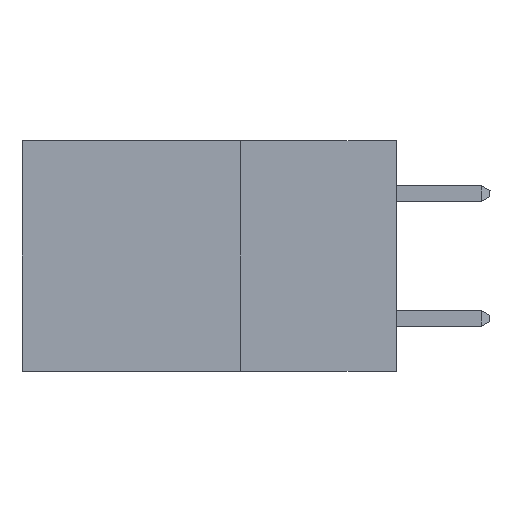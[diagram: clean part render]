
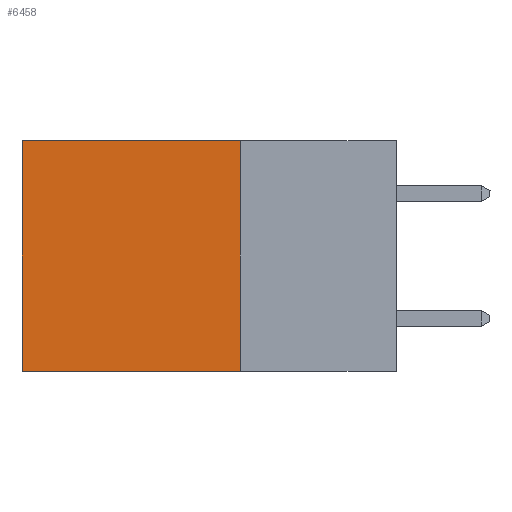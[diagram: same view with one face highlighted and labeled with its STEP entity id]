
A CAD part, left-side view. The second image highlights one B-rep face of the part: STEP entity #6458.
In plain terms, the highlighted planar face has unit normal (-1, 0, 0).
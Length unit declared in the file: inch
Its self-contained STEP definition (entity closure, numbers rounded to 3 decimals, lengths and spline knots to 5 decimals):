
#455 = ORIENTED_EDGE ( 'NONE', *, *, #11606, .F. ) ;
#630 = CARTESIAN_POINT ( 'NONE',  ( 0.298, 0.6, 0. ) ) ;
#826 = LINE ( 'NONE', #5693, #5773 ) ;
#898 = DIRECTION ( 'NONE',  ( 0., 1., 0. ) ) ;
#915 = ORIENTED_EDGE ( 'NONE', *, *, #4939, .F. ) ;
#1008 = VECTOR ( 'NONE', #10337, 39.37008 ) ;
#1098 = CARTESIAN_POINT ( 'NONE',  ( 0.298, 0.25, -0.37 ) ) ;
#1329 = LINE ( 'NONE', #3199, #1008 ) ;
#1333 = VERTEX_POINT ( 'NONE', #630 ) ;
#1512 = EDGE_LOOP ( 'NONE', ( #10101, #915, #455, #8527 ) ) ;
#2091 = VERTEX_POINT ( 'NONE', #1098 ) ;
#2279 = DIRECTION ( 'NONE',  ( 0., 0., -1. ) ) ;
#2392 = VECTOR ( 'NONE', #898, 39.37008 ) ;
#3199 = CARTESIAN_POINT ( 'NONE',  ( 0.298, 0.25, -0.37 ) ) ;
#3683 = PLANE ( 'NONE',  #12043 ) ;
#4611 = FACE_OUTER_BOUND ( 'NONE', #1512, .T. ) ;
#4798 = DIRECTION ( 'NONE',  ( 1., 0., 0. ) ) ;
#4931 = CARTESIAN_POINT ( 'NONE',  ( 0.298, 0.6, -0.37 ) ) ;
#4939 = EDGE_CURVE ( 'NONE', #2091, #11762, #1329, .T. ) ;
#4987 = LINE ( 'NONE', #9526, #10041 ) ;
#5693 = CARTESIAN_POINT ( 'NONE',  ( 0.298, 0.25, 0. ) ) ;
#5773 = VECTOR ( 'NONE', #6757, 39.37008 ) ;
#6458 = ADVANCED_FACE ( 'NONE', ( #4611 ), #3683, .F. ) ;
#6757 = DIRECTION ( 'NONE',  ( 0., 0., -1. ) ) ;
#7278 = EDGE_CURVE ( 'NONE', #8865, #1333, #13086, .T. ) ;
#8527 = ORIENTED_EDGE ( 'NONE', *, *, #7278, .T. ) ;
#8865 = VERTEX_POINT ( 'NONE', #9632 ) ;
#9526 = CARTESIAN_POINT ( 'NONE',  ( 0.298, 0.6, 0. ) ) ;
#9632 = CARTESIAN_POINT ( 'NONE',  ( 0.298, 0.25, 0. ) ) ;
#10041 = VECTOR ( 'NONE', #2279, 39.37008 ) ;
#10101 = ORIENTED_EDGE ( 'NONE', *, *, #12099, .T. ) ;
#10337 = DIRECTION ( 'NONE',  ( 0., 1., 0. ) ) ;
#10807 = CARTESIAN_POINT ( 'NONE',  ( 0.298, 0.25, 0. ) ) ;
#11112 = CARTESIAN_POINT ( 'NONE',  ( 0.298, 0.25, 0. ) ) ;
#11606 = EDGE_CURVE ( 'NONE', #8865, #2091, #826, .T. ) ;
#11762 = VERTEX_POINT ( 'NONE', #4931 ) ;
#11763 = DIRECTION ( 'NONE',  ( 0., 0., -1. ) ) ;
#12043 = AXIS2_PLACEMENT_3D ( 'NONE', #10807, #4798, #11763 ) ;
#12099 = EDGE_CURVE ( 'NONE', #1333, #11762, #4987, .T. ) ;
#13086 = LINE ( 'NONE', #11112, #2392 ) ;
